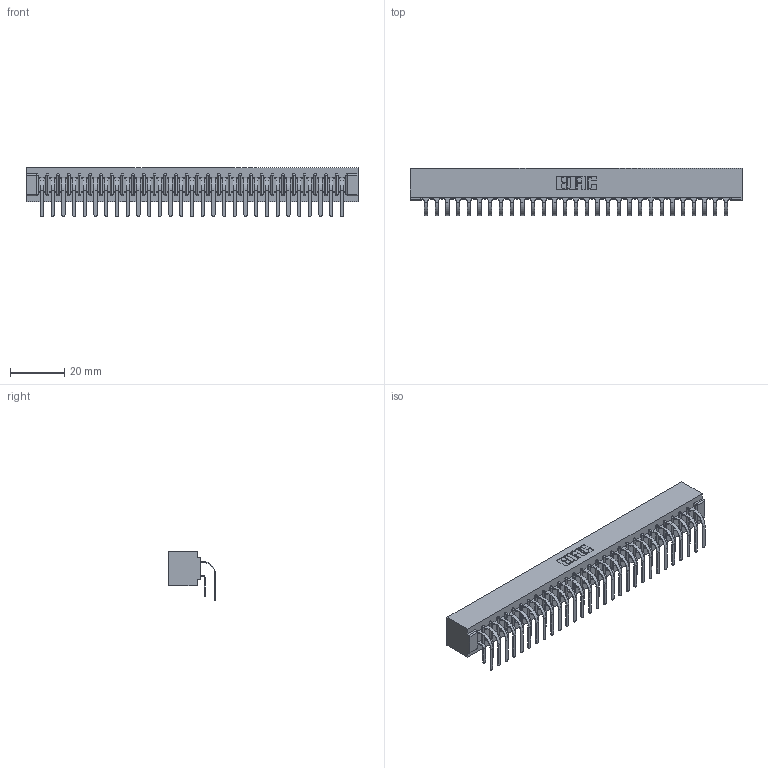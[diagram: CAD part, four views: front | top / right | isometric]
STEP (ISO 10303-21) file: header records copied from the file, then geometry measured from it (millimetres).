
FILE_DESCRIPTION (( 'STEP AP203' ), '1' );
FILE_NAME ('357-058-559-201.STEP', '2022-07-08T22:01:25', ( '' ), ( '' ), 'SwSTEP 2.0', 'SolidWorks 2020', '' );
FILE_SCHEMA (( 'CONFIG_CONTROL_DESIGN' ));
Length unit declared in the file: inch
Products named in the file (4): 307-290-001_558 559 - 1 (Single); 307 Part_No Mounting Lugs; 357-058-559-201; 307-290-001_559 - 2 (Single)
Assembly tree (59 placements, depth 2):
  357-058-559-201
    307 Part_No Mounting Lugs
    307-290-001_558 559 - 1 (Single)  x29
    307-290-001_559 - 2 (Single)  x29
Bounding box: 122.78 x 17.51 x 18.07 mm (x, y, z)
Volume: 13730.2 mm3; surface area: 18095 mm2
Topology: 59 solids, 59 shells, 3040 faces, 8535 edges, 5530 vertices
Faces by surface type: plane 1980, cylinder 1000, sphere 60
Entity records: 28561 total; most frequent: CARTESIAN_POINT 4675, ORIENTED_EDGE 4630, DIRECTION 4583, EDGE_CURVE 2315, VECTOR 1771, LINE 1771, VERTEX_POINT 1498, AXIS2_PLACEMENT_3D 1406
